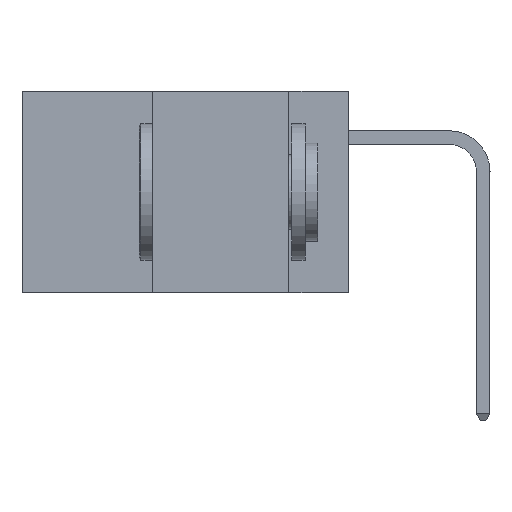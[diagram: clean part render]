
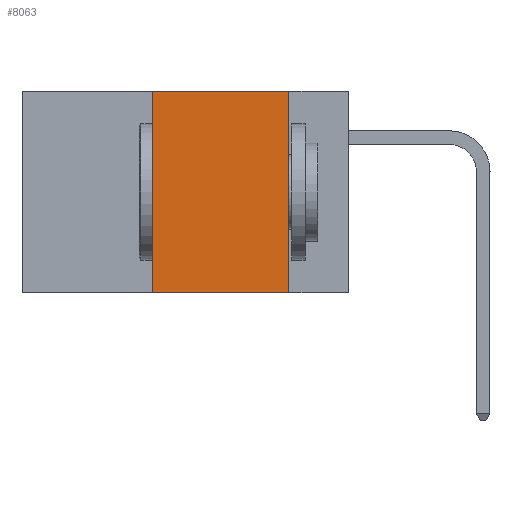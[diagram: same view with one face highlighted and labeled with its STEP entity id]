
A CAD part, left-side view. The second image highlights one B-rep face of the part: STEP entity #8063.
In plain terms, the highlighted planar face has unit normal (-1, 0, 0).
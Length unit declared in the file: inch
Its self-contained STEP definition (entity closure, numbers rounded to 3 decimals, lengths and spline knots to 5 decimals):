
#149 = AXIS2_PLACEMENT_3D ( 'NONE', #6191, #8445, #2507 ) ;
#350 = CARTESIAN_POINT ( 'NONE',  ( 0., 0.11, 0. ) ) ;
#396 = ORIENTED_EDGE ( 'NONE', *, *, #8811, .F. ) ;
#1018 = VERTEX_POINT ( 'NONE', #2731 ) ;
#1086 = VERTEX_POINT ( 'NONE', #1554 ) ;
#1104 = CARTESIAN_POINT ( 'NONE',  ( 0., 0.11, 0. ) ) ;
#1244 = CARTESIAN_POINT ( 'NONE',  ( 0., 0.36, 0. ) ) ;
#1554 = CARTESIAN_POINT ( 'NONE',  ( 0., 0.11, -0.37 ) ) ;
#1782 = LINE ( 'NONE', #1104, #9208 ) ;
#2221 = VECTOR ( 'NONE', #5665, 39.37008 ) ;
#2447 = LINE ( 'NONE', #9394, #4385 ) ;
#2507 = DIRECTION ( 'NONE',  ( 0., 0., -1. ) ) ;
#2731 = CARTESIAN_POINT ( 'NONE',  ( 0., 0.36, 0. ) ) ;
#2877 = EDGE_CURVE ( 'NONE', #1018, #4112, #5259, .T. ) ;
#3739 = CARTESIAN_POINT ( 'NONE',  ( 0., 0.36, -0.37 ) ) ;
#4112 = VERTEX_POINT ( 'NONE', #350 ) ;
#4175 = DIRECTION ( 'NONE',  ( 0., -1., 0. ) ) ;
#4382 = LINE ( 'NONE', #1244, #2221 ) ;
#4385 = VECTOR ( 'NONE', #4175, 39.37008 ) ;
#5259 = LINE ( 'NONE', #6270, #8552 ) ;
#5509 = DIRECTION ( 'NONE',  ( 0., -1., 0. ) ) ;
#5524 = DIRECTION ( 'NONE',  ( 0., 0., -1. ) ) ;
#5594 = ORIENTED_EDGE ( 'NONE', *, *, #2877, .F. ) ;
#5596 = EDGE_CURVE ( 'NONE', #7037, #1018, #4382, .T. ) ;
#5665 = DIRECTION ( 'NONE',  ( 0., 0., 1. ) ) ;
#6191 = CARTESIAN_POINT ( 'NONE',  ( 0., 0.6, 0. ) ) ;
#6270 = CARTESIAN_POINT ( 'NONE',  ( 0., 0.6, 0. ) ) ;
#6625 = EDGE_LOOP ( 'NONE', ( #396, #5594, #9341, #8894 ) ) ;
#6970 = PLANE ( 'NONE',  #149 ) ;
#7037 = VERTEX_POINT ( 'NONE', #3739 ) ;
#8063 = ADVANCED_FACE ( 'NONE', ( #8083 ), #6970, .F. ) ;
#8083 = FACE_OUTER_BOUND ( 'NONE', #6625, .T. ) ;
#8445 = DIRECTION ( 'NONE',  ( 1., 0., 0. ) ) ;
#8552 = VECTOR ( 'NONE', #5509, 39.37008 ) ;
#8811 = EDGE_CURVE ( 'NONE', #4112, #1086, #1782, .T. ) ;
#8894 = ORIENTED_EDGE ( 'NONE', *, *, #9577, .T. ) ;
#9208 = VECTOR ( 'NONE', #5524, 39.37008 ) ;
#9341 = ORIENTED_EDGE ( 'NONE', *, *, #5596, .F. ) ;
#9394 = CARTESIAN_POINT ( 'NONE',  ( 0., 0.6, -0.37 ) ) ;
#9577 = EDGE_CURVE ( 'NONE', #7037, #1086, #2447, .T. ) ;
